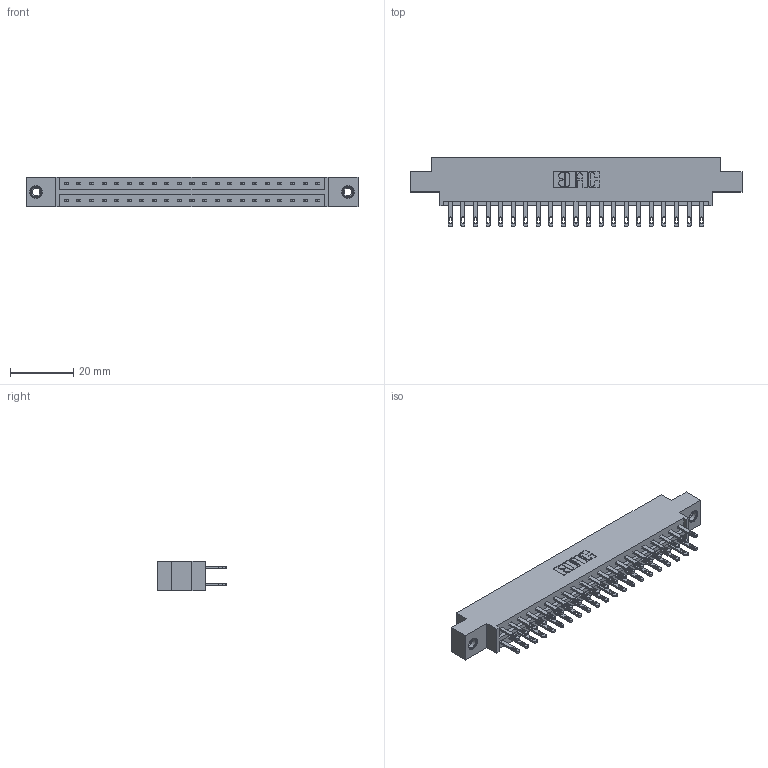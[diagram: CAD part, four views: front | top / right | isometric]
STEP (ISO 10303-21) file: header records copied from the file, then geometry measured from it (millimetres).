
FILE_DESCRIPTION (( 'STEP AP203' ), '1' );
FILE_NAME ('333-042-500-807.STEP', '2018-08-03T16:01:07', ( '' ), ( '' ), 'SwSTEP 2.0', 'SolidWorks 2016', '' );
FILE_SCHEMA (( 'CONFIG_CONTROL_DESIGN' ));
Length unit declared in the file: inch
Products named in the file (4): 333 Part_Offset - .156 Dia - TI; 345-292-001_345-293-100; 345-250-001_345-250-005-103; 333-042-500-807
Assembly tree (45 placements, depth 2):
  333-042-500-807
    333 Part_Offset - .156 Dia - TI
    345-292-001_345-293-100  x42
    345-250-001_345-250-005-103  x2
Bounding box: 104.75 x 21.85 x 9.4 mm (x, y, z)
Volume: 10385 mm3; surface area: 12769.1 mm2
Topology: 45 solids, 45 shells, 2194 faces, 6633 edges, 4414 vertices
Faces by surface type: plane 1366, cylinder 812, cone 12, torus 4
Entity records: 17474 total; most frequent: CARTESIAN_POINT 2905, ORIENTED_EDGE 2834, DIRECTION 2551, EDGE_CURVE 1417, LINE 1265, VECTOR 1265, VERTEX_POINT 940, AXIS2_PLACEMENT_3D 643
